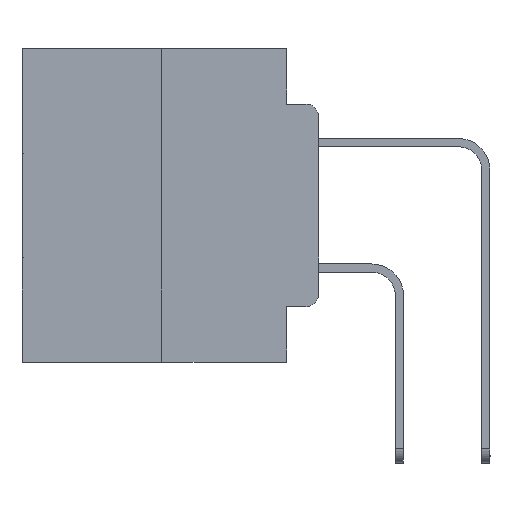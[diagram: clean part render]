
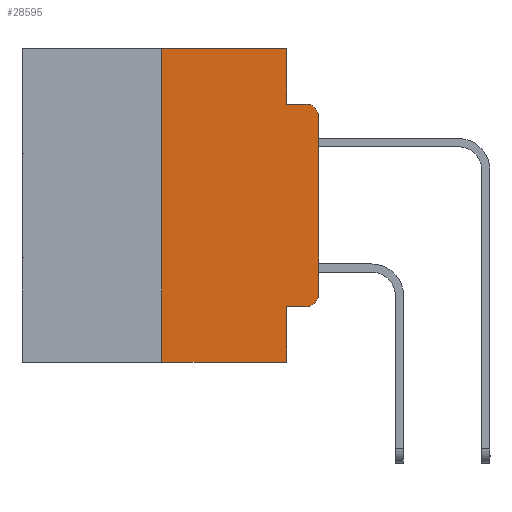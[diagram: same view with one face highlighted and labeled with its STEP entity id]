
A CAD part, left-side view. The second image highlights one B-rep face of the part: STEP entity #28595.
In plain terms, the highlighted planar face has unit normal (-1, 0, 0).
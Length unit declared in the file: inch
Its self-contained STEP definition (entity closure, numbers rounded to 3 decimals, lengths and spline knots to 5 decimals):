
#61 = VERTEX_POINT ( 'NONE', #10950 ) ;
#1272 = CARTESIAN_POINT ( 'NONE',  ( 0., 0.051, -0.5 ) ) ;
#1384 = LINE ( 'NONE', #11616, #31515 ) ;
#1930 = ORIENTED_EDGE ( 'NONE', *, *, #17910, .T. ) ;
#2001 = DIRECTION ( 'NONE',  ( 0., 0., -1. ) ) ;
#2464 = EDGE_LOOP ( 'NONE', ( #1930, #19204, #14952, #21448, #13929, #12335, #11795, #22300, #9873, #27198 ) ) ;
#2907 = DIRECTION ( 'NONE',  ( 0., -1., 0. ) ) ;
#2962 = DIRECTION ( 'NONE',  ( 0., -1., 0. ) ) ;
#2971 = DIRECTION ( 'NONE',  ( -1., 0., 0. ) ) ;
#3611 = CARTESIAN_POINT ( 'NONE',  ( 0., 0., 0. ) ) ;
#3797 = EDGE_CURVE ( 'NONE', #16806, #9397, #27074, .T. ) ;
#3840 = EDGE_CURVE ( 'NONE', #24883, #15037, #13775, .T. ) ;
#3863 = VECTOR ( 'NONE', #2962, 39.37008 ) ;
#4522 = EDGE_CURVE ( 'NONE', #24883, #17551, #24001, .T. ) ;
#5789 = CARTESIAN_POINT ( 'NONE',  ( 0., 0.051, -0.4115 ) ) ;
#6076 = DIRECTION ( 'NONE',  ( 0., 0., -1. ) ) ;
#6187 = CARTESIAN_POINT ( 'NONE',  ( 0., 0.051, 0. ) ) ;
#6589 = VERTEX_POINT ( 'NONE', #14464 ) ;
#6633 = EDGE_CURVE ( 'NONE', #9397, #27875, #1384, .T. ) ;
#7183 = AXIS2_PLACEMENT_3D ( 'NONE', #14199, #26535, #17285 ) ;
#9397 = VERTEX_POINT ( 'NONE', #24511 ) ;
#9566 = CARTESIAN_POINT ( 'NONE',  ( 0., 0.25, 0. ) ) ;
#9606 = EDGE_CURVE ( 'NONE', #27875, #6589, #24904, .T. ) ;
#9873 = ORIENTED_EDGE ( 'NONE', *, *, #4522, .T. ) ;
#9932 = CARTESIAN_POINT ( 'NONE',  ( 0., 0.25, -0.5 ) ) ;
#10638 = CARTESIAN_POINT ( 'NONE',  ( 0., 0.051, -0.0885 ) ) ;
#10950 = CARTESIAN_POINT ( 'NONE',  ( 0., 0., -0.1085 ) ) ;
#10954 = DIRECTION ( 'NONE',  ( 0., 0., 1. ) ) ;
#11616 = CARTESIAN_POINT ( 'NONE',  ( 0., 0.051, 0. ) ) ;
#11673 = CARTESIAN_POINT ( 'NONE',  ( 0., 0.051, -0.0885 ) ) ;
#11795 = ORIENTED_EDGE ( 'NONE', *, *, #29354, .T. ) ;
#11957 = VECTOR ( 'NONE', #12584, 39.37008 ) ;
#12335 = ORIENTED_EDGE ( 'NONE', *, *, #22833, .F. ) ;
#12584 = DIRECTION ( 'NONE',  ( 0., -1., 0. ) ) ;
#13001 = VECTOR ( 'NONE', #30471, 39.37008 ) ;
#13245 = VERTEX_POINT ( 'NONE', #15571 ) ;
#13513 = CIRCLE ( 'NONE', #24204, 0.02 ) ;
#13775 = LINE ( 'NONE', #6187, #13001 ) ;
#13852 = CARTESIAN_POINT ( 'NONE',  ( 0., 0.051, -0.4115 ) ) ;
#13929 = ORIENTED_EDGE ( 'NONE', *, *, #3797, .F. ) ;
#14199 = CARTESIAN_POINT ( 'NONE',  ( 0., 0.473, 0. ) ) ;
#14464 = CARTESIAN_POINT ( 'NONE',  ( 0., 0.02, -0.0885 ) ) ;
#14510 = PLANE ( 'NONE',  #7183 ) ;
#14952 = ORIENTED_EDGE ( 'NONE', *, *, #9606, .F. ) ;
#15037 = VERTEX_POINT ( 'NONE', #1272 ) ;
#15418 = CARTESIAN_POINT ( 'NONE',  ( 0., 0.02, -0.4115 ) ) ;
#15571 = CARTESIAN_POINT ( 'NONE',  ( 0., 0., -0.3915 ) ) ;
#16806 = VERTEX_POINT ( 'NONE', #29849 ) ;
#17285 = DIRECTION ( 'NONE',  ( 0., 0., -1. ) ) ;
#17551 = VERTEX_POINT ( 'NONE', #15418 ) ;
#17613 = VECTOR ( 'NONE', #10954, 39.37008 ) ;
#17768 = CARTESIAN_POINT ( 'NONE',  ( 0., 0.02, -0.3915 ) ) ;
#17910 = EDGE_CURVE ( 'NONE', #13245, #61, #27130, .T. ) ;
#19204 = ORIENTED_EDGE ( 'NONE', *, *, #22577, .T. ) ;
#20183 = VECTOR ( 'NONE', #23839, 39.37008 ) ;
#21448 = ORIENTED_EDGE ( 'NONE', *, *, #6633, .F. ) ;
#21493 = VECTOR ( 'NONE', #28759, 39.37008 ) ;
#22026 = CARTESIAN_POINT ( 'NONE',  ( 0., 0.473, -0.5 ) ) ;
#22087 = AXIS2_PLACEMENT_3D ( 'NONE', #17768, #2971, #24914 ) ;
#22300 = ORIENTED_EDGE ( 'NONE', *, *, #3840, .F. ) ;
#22577 = EDGE_CURVE ( 'NONE', #61, #6589, #13513, .T. ) ;
#22833 = EDGE_CURVE ( 'NONE', #28641, #16806, #27962, .T. ) ;
#23741 = FACE_OUTER_BOUND ( 'NONE', #2464, .T. ) ;
#23839 = DIRECTION ( 'NONE',  ( 0., -1., 0. ) ) ;
#24001 = LINE ( 'NONE', #13852, #20183 ) ;
#24204 = AXIS2_PLACEMENT_3D ( 'NONE', #28023, #25253, #6076 ) ;
#24438 = VECTOR ( 'NONE', #2907, 39.37008 ) ;
#24511 = CARTESIAN_POINT ( 'NONE',  ( 0., 0.051, 0. ) ) ;
#24883 = VERTEX_POINT ( 'NONE', #5789 ) ;
#24904 = LINE ( 'NONE', #10638, #11957 ) ;
#24914 = DIRECTION ( 'NONE',  ( 0., 0., -1. ) ) ;
#25253 = DIRECTION ( 'NONE',  ( -1., 0., 0. ) ) ;
#26535 = DIRECTION ( 'NONE',  ( 1., 0., 0. ) ) ;
#27074 = LINE ( 'NONE', #27483, #24438 ) ;
#27130 = LINE ( 'NONE', #3611, #17613 ) ;
#27198 = ORIENTED_EDGE ( 'NONE', *, *, #30822, .T. ) ;
#27483 = CARTESIAN_POINT ( 'NONE',  ( 0., 0.473, 0. ) ) ;
#27875 = VERTEX_POINT ( 'NONE', #11673 ) ;
#27962 = LINE ( 'NONE', #9566, #21493 ) ;
#28023 = CARTESIAN_POINT ( 'NONE',  ( 0., 0.02, -0.1085 ) ) ;
#28595 = ADVANCED_FACE ( 'NONE', ( #23741 ), #14510, .F. ) ;
#28641 = VERTEX_POINT ( 'NONE', #9932 ) ;
#28759 = DIRECTION ( 'NONE',  ( 0., 0., 1. ) ) ;
#29354 = EDGE_CURVE ( 'NONE', #28641, #15037, #30534, .T. ) ;
#29849 = CARTESIAN_POINT ( 'NONE',  ( 0., 0.25, 0. ) ) ;
#30446 = CIRCLE ( 'NONE', #22087, 0.02 ) ;
#30471 = DIRECTION ( 'NONE',  ( 0., 0., -1. ) ) ;
#30534 = LINE ( 'NONE', #22026, #3863 ) ;
#30822 = EDGE_CURVE ( 'NONE', #17551, #13245, #30446, .T. ) ;
#31515 = VECTOR ( 'NONE', #2001, 39.37008 ) ;
